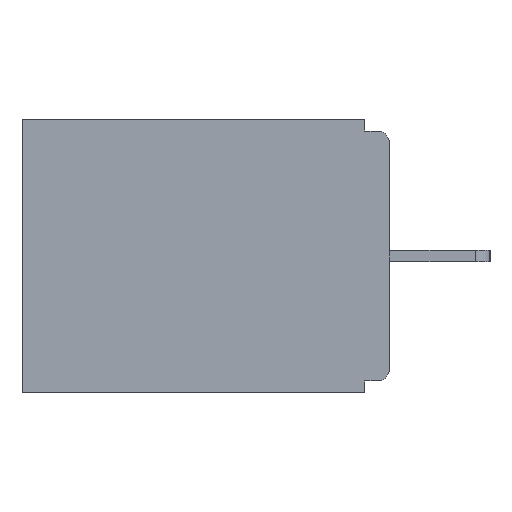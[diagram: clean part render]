
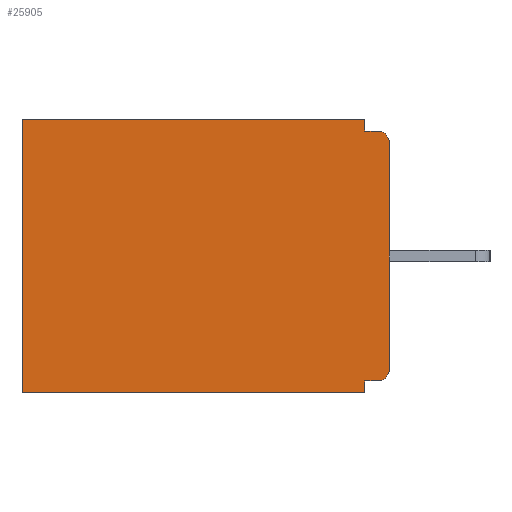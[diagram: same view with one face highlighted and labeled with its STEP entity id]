
A CAD part, left-side view. The second image highlights one B-rep face of the part: STEP entity #25905.
In plain terms, the highlighted planar face has unit normal (-1, 0, 0).
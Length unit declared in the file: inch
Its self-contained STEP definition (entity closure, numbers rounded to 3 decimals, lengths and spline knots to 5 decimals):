
#105 = DIRECTION ( 'NONE',  ( 0., 0., -1. ) ) ;
#183 = DIRECTION ( 'NONE',  ( 1., 0., 0. ) ) ;
#198 = VERTEX_POINT ( 'NONE', #25444 ) ;
#890 = AXIS2_PLACEMENT_3D ( 'NONE', #10734, #183, #14944 ) ;
#933 = VECTOR ( 'NONE', #13649, 39.37008 ) ;
#1438 = VERTEX_POINT ( 'NONE', #13939 ) ;
#1995 = DIRECTION ( 'NONE',  ( 0., 0., -1. ) ) ;
#2492 = ORIENTED_EDGE ( 'NONE', *, *, #13194, .T. ) ;
#4605 = VECTOR ( 'NONE', #6643, 39.37008 ) ;
#4936 = VERTEX_POINT ( 'NONE', #24002 ) ;
#5005 = VERTEX_POINT ( 'NONE', #24268 ) ;
#5127 = EDGE_CURVE ( 'NONE', #5005, #6110, #6570, .T. ) ;
#5691 = EDGE_CURVE ( 'NONE', #22411, #1438, #14431, .T. ) ;
#6016 = ORIENTED_EDGE ( 'NONE', *, *, #22424, .T. ) ;
#6070 = CARTESIAN_POINT ( 'NONE',  ( 0.298, 0.031, -0.328 ) ) ;
#6110 = VERTEX_POINT ( 'NONE', #8111 ) ;
#6570 = LINE ( 'NONE', #13682, #933 ) ;
#6643 = DIRECTION ( 'NONE',  ( 0., 0., -1. ) ) ;
#6980 = CARTESIAN_POINT ( 'NONE',  ( 0.298, 0.46, 0. ) ) ;
#7267 = EDGE_CURVE ( 'NONE', #4936, #9767, #20668, .T. ) ;
#7342 = CIRCLE ( 'NONE', #10210, 0.015 ) ;
#7529 = VECTOR ( 'NONE', #9068, 39.37008 ) ;
#7784 = CARTESIAN_POINT ( 'NONE',  ( 0.298, 0.015, -0.015 ) ) ;
#8111 = CARTESIAN_POINT ( 'NONE',  ( 0.298, 0.46, -0.343 ) ) ;
#8420 = VECTOR ( 'NONE', #9962, 39.37008 ) ;
#8537 = CARTESIAN_POINT ( 'NONE',  ( 0.298, 0.46, 0. ) ) ;
#8781 = DIRECTION ( 'NONE',  ( -1., 0., 0. ) ) ;
#9068 = DIRECTION ( 'NONE',  ( 0., -1., 0. ) ) ;
#9102 = CARTESIAN_POINT ( 'NONE',  ( 0.298, 0., -0.015 ) ) ;
#9629 = VECTOR ( 'NONE', #105, 39.37008 ) ;
#9766 = CIRCLE ( 'NONE', #18289, 0.015 ) ;
#9767 = VERTEX_POINT ( 'NONE', #6070 ) ;
#9962 = DIRECTION ( 'NONE',  ( 0., 1., 0. ) ) ;
#10210 = AXIS2_PLACEMENT_3D ( 'NONE', #26683, #14607, #1995 ) ;
#10506 = CARTESIAN_POINT ( 'NONE',  ( 0.298, 0.031, -0.343 ) ) ;
#10648 = CARTESIAN_POINT ( 'NONE',  ( 0.298, 0., -0.328 ) ) ;
#10734 = CARTESIAN_POINT ( 'NONE',  ( 0.298, 0., 0. ) ) ;
#11391 = EDGE_LOOP ( 'NONE', ( #18496, #25261, #23712, #6016, #11669, #26276, #19959, #19679, #2492, #22081 ) ) ;
#11541 = DIRECTION ( 'NONE',  ( 0., 1., 0. ) ) ;
#11669 = ORIENTED_EDGE ( 'NONE', *, *, #21633, .T. ) ;
#12148 = EDGE_CURVE ( 'NONE', #23672, #18271, #23954, .T. ) ;
#12969 = FACE_OUTER_BOUND ( 'NONE', #11391, .T. ) ;
#13194 = EDGE_CURVE ( 'NONE', #4936, #1438, #9766, .T. ) ;
#13558 = CARTESIAN_POINT ( 'NONE',  ( 0.298, 0., 0. ) ) ;
#13649 = DIRECTION ( 'NONE',  ( 0., 1., 0. ) ) ;
#13682 = CARTESIAN_POINT ( 'NONE',  ( 0.298, 0., -0.343 ) ) ;
#13722 = EDGE_CURVE ( 'NONE', #9767, #5005, #23549, .T. ) ;
#13939 = CARTESIAN_POINT ( 'NONE',  ( 0.298, 0., -0.313 ) ) ;
#14431 = LINE ( 'NONE', #20305, #19811 ) ;
#14607 = DIRECTION ( 'NONE',  ( -1., 0., 0. ) ) ;
#14944 = DIRECTION ( 'NONE',  ( 0., 0., -1. ) ) ;
#15112 = VECTOR ( 'NONE', #11541, 39.37008 ) ;
#15175 = LINE ( 'NONE', #8537, #9629 ) ;
#15610 = CARTESIAN_POINT ( 'NONE',  ( 0.298, 0., -0.03 ) ) ;
#15712 = LINE ( 'NONE', #18942, #4605 ) ;
#16840 = PLANE ( 'NONE',  #890 ) ;
#18271 = VERTEX_POINT ( 'NONE', #7784 ) ;
#18289 = AXIS2_PLACEMENT_3D ( 'NONE', #21115, #8781, #23181 ) ;
#18496 = ORIENTED_EDGE ( 'NONE', *, *, #21553, .T. ) ;
#18942 = CARTESIAN_POINT ( 'NONE',  ( 0.298, 0.031, -0.343 ) ) ;
#19388 = VECTOR ( 'NONE', #24871, 39.37008 ) ;
#19679 = ORIENTED_EDGE ( 'NONE', *, *, #7267, .F. ) ;
#19811 = VECTOR ( 'NONE', #21558, 39.37008 ) ;
#19959 = ORIENTED_EDGE ( 'NONE', *, *, #13722, .F. ) ;
#20305 = CARTESIAN_POINT ( 'NONE',  ( 0.298, 0., 0. ) ) ;
#20668 = LINE ( 'NONE', #10648, #8420 ) ;
#21115 = CARTESIAN_POINT ( 'NONE',  ( 0.298, 0.015, -0.313 ) ) ;
#21149 = LINE ( 'NONE', #13558, #15112 ) ;
#21553 = EDGE_CURVE ( 'NONE', #22411, #18271, #7342, .T. ) ;
#21558 = DIRECTION ( 'NONE',  ( 0., 0., -1. ) ) ;
#21633 = EDGE_CURVE ( 'NONE', #23582, #6110, #15175, .T. ) ;
#22081 = ORIENTED_EDGE ( 'NONE', *, *, #5691, .F. ) ;
#22411 = VERTEX_POINT ( 'NONE', #15610 ) ;
#22424 = EDGE_CURVE ( 'NONE', #198, #23582, #21149, .T. ) ;
#22852 = EDGE_CURVE ( 'NONE', #198, #23672, #15712, .T. ) ;
#23181 = DIRECTION ( 'NONE',  ( 0., 0., -1. ) ) ;
#23549 = LINE ( 'NONE', #10506, #19388 ) ;
#23582 = VERTEX_POINT ( 'NONE', #6980 ) ;
#23672 = VERTEX_POINT ( 'NONE', #23737 ) ;
#23712 = ORIENTED_EDGE ( 'NONE', *, *, #22852, .F. ) ;
#23737 = CARTESIAN_POINT ( 'NONE',  ( 0.298, 0.031, -0.015 ) ) ;
#23954 = LINE ( 'NONE', #9102, #7529 ) ;
#24002 = CARTESIAN_POINT ( 'NONE',  ( 0.298, 0.015, -0.328 ) ) ;
#24268 = CARTESIAN_POINT ( 'NONE',  ( 0.298, 0.031, -0.343 ) ) ;
#24871 = DIRECTION ( 'NONE',  ( 0., 0., -1. ) ) ;
#25261 = ORIENTED_EDGE ( 'NONE', *, *, #12148, .F. ) ;
#25444 = CARTESIAN_POINT ( 'NONE',  ( 0.298, 0.031, 0. ) ) ;
#25905 = ADVANCED_FACE ( 'NONE', ( #12969 ), #16840, .F. ) ;
#26276 = ORIENTED_EDGE ( 'NONE', *, *, #5127, .F. ) ;
#26683 = CARTESIAN_POINT ( 'NONE',  ( 0.298, 0.015, -0.03 ) ) ;
